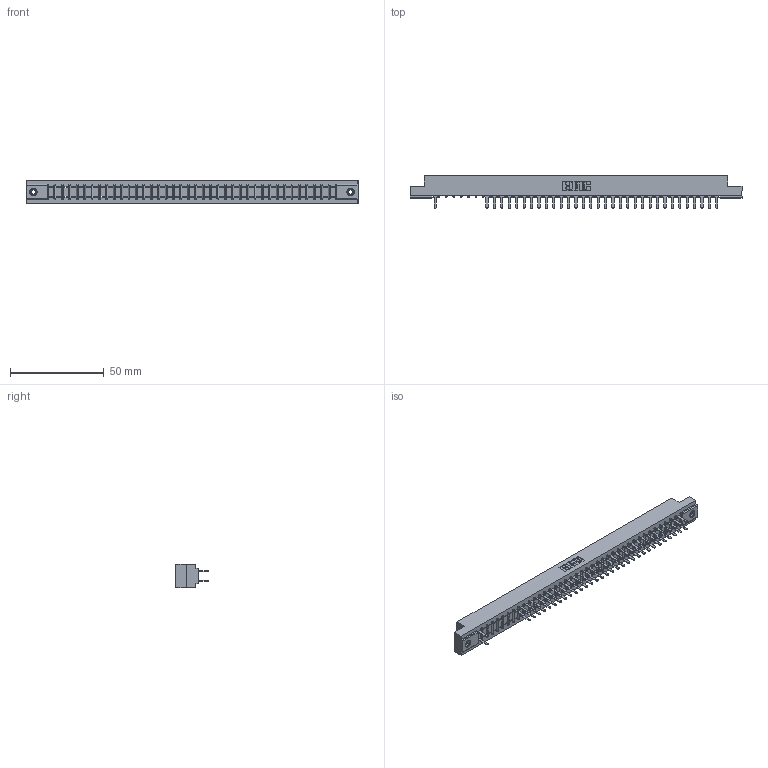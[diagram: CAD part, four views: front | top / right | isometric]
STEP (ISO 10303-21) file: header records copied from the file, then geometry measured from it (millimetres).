
FILE_DESCRIPTION (( 'STEP AP203' ), '1' );
FILE_NAME ('307-078-520-208.STEP', '2018-08-06T17:31:06', ( '' ), ( '' ), 'SwSTEP 2.0', 'SolidWorks 2016', '' );
FILE_SCHEMA (( 'CONFIG_CONTROL_DESIGN' ));
Length unit declared in the file: inch
Products named in the file (4): 307 Part_.156 Dia Mounting Holes; 307-290-001_520; 345-250-001_345-250-003-102; 307-078-520-208
Assembly tree (68 placements, depth 2):
  307-078-520-208
    307 Part_.156 Dia Mounting Holes
    307-290-001_520  x65
    345-250-001_345-250-003-102  x2
Bounding box: 177.55 x 17.42 x 12.7 mm (x, y, z)
Volume: 18731.5 mm3; surface area: 21878.2 mm2
Topology: 68 solids, 68 shells, 3338 faces, 9325 edges, 6014 vertices
Faces by surface type: plane 2195, cylinder 1047, sphere 80, cone 12, torus 4
Entity records: 35789 total; most frequent: CARTESIAN_POINT 5893, ORIENTED_EDGE 5846, DIRECTION 5769, EDGE_CURVE 2923, VECTOR 2241, LINE 2241, VERTEX_POINT 1888, AXIS2_PLACEMENT_3D 1764
